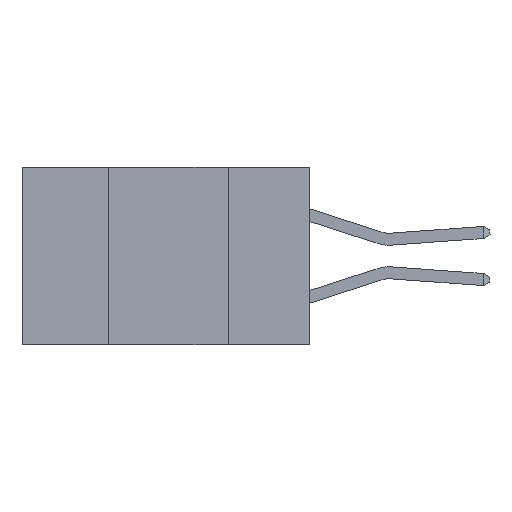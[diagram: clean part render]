
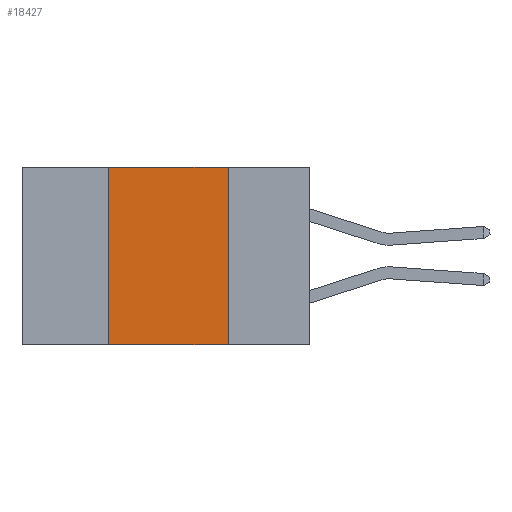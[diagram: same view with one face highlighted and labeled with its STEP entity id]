
A CAD part, left-side view. The second image highlights one B-rep face of the part: STEP entity #18427.
In plain terms, the highlighted planar face has unit normal (-1, 0, 0).
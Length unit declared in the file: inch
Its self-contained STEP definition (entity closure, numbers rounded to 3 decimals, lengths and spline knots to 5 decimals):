
#127 = LINE ( 'NONE', #19400, #15023 ) ;
#786 = DIRECTION ( 'NONE',  ( 0., -1., 0. ) ) ;
#920 = VECTOR ( 'NONE', #1985, 39.37008 ) ;
#989 = CARTESIAN_POINT ( 'NONE',  ( 0., 0.17, 0. ) ) ;
#1524 = FACE_OUTER_BOUND ( 'NONE', #16948, .T. ) ;
#1985 = DIRECTION ( 'NONE',  ( 0., 0., 1. ) ) ;
#2770 = LINE ( 'NONE', #18762, #17625 ) ;
#2789 = VERTEX_POINT ( 'NONE', #989 ) ;
#2973 = ORIENTED_EDGE ( 'NONE', *, *, #10691, .F. ) ;
#3865 = PLANE ( 'NONE',  #18047 ) ;
#4893 = VECTOR ( 'NONE', #786, 39.37008 ) ;
#5868 = CARTESIAN_POINT ( 'NONE',  ( 0., 0.42, 0. ) ) ;
#7811 = DIRECTION ( 'NONE',  ( 0., 0., -1. ) ) ;
#8769 = ORIENTED_EDGE ( 'NONE', *, *, #23120, .F. ) ;
#10056 = LINE ( 'NONE', #14382, #4893 ) ;
#10518 = CARTESIAN_POINT ( 'NONE',  ( 0., 0.42, -0.37 ) ) ;
#10691 = EDGE_CURVE ( 'NONE', #2789, #23973, #2770, .T. ) ;
#10982 = CARTESIAN_POINT ( 'NONE',  ( 0., 0.17, -0.37 ) ) ;
#13558 = VERTEX_POINT ( 'NONE', #14380 ) ;
#13925 = ORIENTED_EDGE ( 'NONE', *, *, #18432, .F. ) ;
#14380 = CARTESIAN_POINT ( 'NONE',  ( 0., 0.42, 0. ) ) ;
#14382 = CARTESIAN_POINT ( 'NONE',  ( 0., 0.6, 0. ) ) ;
#15023 = VECTOR ( 'NONE', #21290, 39.37008 ) ;
#15378 = EDGE_CURVE ( 'NONE', #22444, #23973, #127, .T. ) ;
#16389 = LINE ( 'NONE', #5868, #920 ) ;
#16948 = EDGE_LOOP ( 'NONE', ( #2973, #8769, #13925, #24667 ) ) ;
#17416 = CARTESIAN_POINT ( 'NONE',  ( 0., 0.6, 0. ) ) ;
#17625 = VECTOR ( 'NONE', #22550, 39.37008 ) ;
#18047 = AXIS2_PLACEMENT_3D ( 'NONE', #17416, #19359, #7811 ) ;
#18427 = ADVANCED_FACE ( 'NONE', ( #1524 ), #3865, .F. ) ;
#18432 = EDGE_CURVE ( 'NONE', #22444, #13558, #16389, .T. ) ;
#18762 = CARTESIAN_POINT ( 'NONE',  ( 0., 0.17, 0. ) ) ;
#19359 = DIRECTION ( 'NONE',  ( 1., 0., 0. ) ) ;
#19400 = CARTESIAN_POINT ( 'NONE',  ( 0., 0.6, -0.37 ) ) ;
#21290 = DIRECTION ( 'NONE',  ( 0., -1., 0. ) ) ;
#22444 = VERTEX_POINT ( 'NONE', #10518 ) ;
#22550 = DIRECTION ( 'NONE',  ( 0., 0., -1. ) ) ;
#23120 = EDGE_CURVE ( 'NONE', #13558, #2789, #10056, .T. ) ;
#23973 = VERTEX_POINT ( 'NONE', #10982 ) ;
#24667 = ORIENTED_EDGE ( 'NONE', *, *, #15378, .T. ) ;
